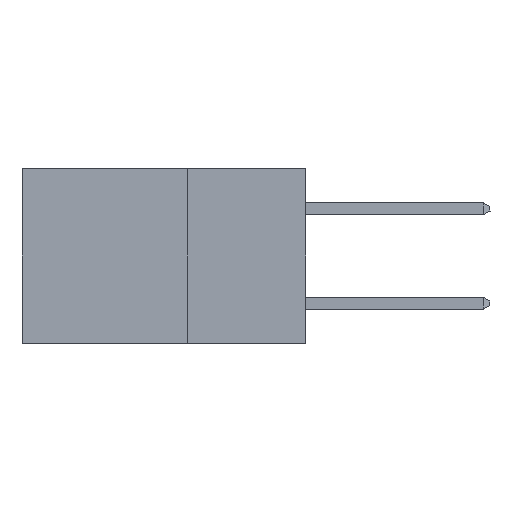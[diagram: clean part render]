
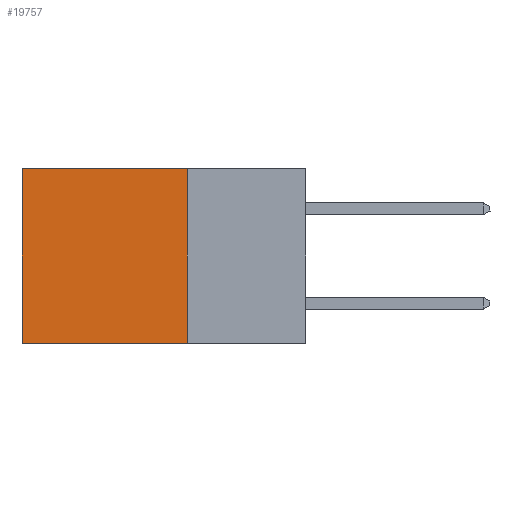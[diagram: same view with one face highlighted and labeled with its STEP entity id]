
A CAD part, left-side view. The second image highlights one B-rep face of the part: STEP entity #19757.
In plain terms, the highlighted planar face has unit normal (-1, 0, 0).
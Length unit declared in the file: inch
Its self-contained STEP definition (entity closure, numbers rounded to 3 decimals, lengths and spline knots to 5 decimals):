
#538 = AXIS2_PLACEMENT_3D ( 'NONE', #612, #7797, #15094 ) ;
#612 = CARTESIAN_POINT ( 'NONE',  ( 0.298, 0.25, 0. ) ) ;
#919 = EDGE_CURVE ( 'NONE', #18641, #7401, #1288, .T. ) ;
#1288 = LINE ( 'NONE', #10321, #15159 ) ;
#1549 = VECTOR ( 'NONE', #2232, 39.37008 ) ;
#2232 = DIRECTION ( 'NONE',  ( 0., 1., 0. ) ) ;
#2436 = PLANE ( 'NONE',  #538 ) ;
#3903 = EDGE_CURVE ( 'NONE', #18641, #4290, #22527, .T. ) ;
#4290 = VERTEX_POINT ( 'NONE', #16801 ) ;
#4875 = ORIENTED_EDGE ( 'NONE', *, *, #11234, .T. ) ;
#7401 = VERTEX_POINT ( 'NONE', #16666 ) ;
#7797 = DIRECTION ( 'NONE',  ( 1., 0., 0. ) ) ;
#8284 = VECTOR ( 'NONE', #14180, 39.37008 ) ;
#8979 = FACE_OUTER_BOUND ( 'NONE', #10619, .T. ) ;
#9746 = CARTESIAN_POINT ( 'NONE',  ( 0.298, 0.6, 0. ) ) ;
#10321 = CARTESIAN_POINT ( 'NONE',  ( 0.298, 0.25, 0. ) ) ;
#10619 = EDGE_LOOP ( 'NONE', ( #4875, #17801, #16601, #12759 ) ) ;
#11234 = EDGE_CURVE ( 'NONE', #4290, #17956, #21867, .T. ) ;
#11471 = DIRECTION ( 'NONE',  ( 0., 0., -1. ) ) ;
#12146 = DIRECTION ( 'NONE',  ( 0., 0., -1. ) ) ;
#12577 = CARTESIAN_POINT ( 'NONE',  ( 0.298, 0.25, -0.37 ) ) ;
#12759 = ORIENTED_EDGE ( 'NONE', *, *, #3903, .T. ) ;
#14180 = DIRECTION ( 'NONE',  ( 0., 1., 0. ) ) ;
#15005 = CARTESIAN_POINT ( 'NONE',  ( 0.298, 0.25, 0. ) ) ;
#15094 = DIRECTION ( 'NONE',  ( 0., 0., -1. ) ) ;
#15159 = VECTOR ( 'NONE', #12146, 39.37008 ) ;
#16601 = ORIENTED_EDGE ( 'NONE', *, *, #919, .F. ) ;
#16666 = CARTESIAN_POINT ( 'NONE',  ( 0.298, 0.25, -0.37 ) ) ;
#16801 = CARTESIAN_POINT ( 'NONE',  ( 0.298, 0.6, 0. ) ) ;
#17801 = ORIENTED_EDGE ( 'NONE', *, *, #22247, .F. ) ;
#17956 = VERTEX_POINT ( 'NONE', #23359 ) ;
#18641 = VERTEX_POINT ( 'NONE', #15005 ) ;
#18753 = VECTOR ( 'NONE', #11471, 39.37008 ) ;
#19757 = ADVANCED_FACE ( 'NONE', ( #8979 ), #2436, .F. ) ;
#20493 = LINE ( 'NONE', #12577, #8284 ) ;
#20601 = CARTESIAN_POINT ( 'NONE',  ( 0.298, 0.25, 0. ) ) ;
#21867 = LINE ( 'NONE', #9746, #18753 ) ;
#22247 = EDGE_CURVE ( 'NONE', #7401, #17956, #20493, .T. ) ;
#22527 = LINE ( 'NONE', #20601, #1549 ) ;
#23359 = CARTESIAN_POINT ( 'NONE',  ( 0.298, 0.6, -0.37 ) ) ;
